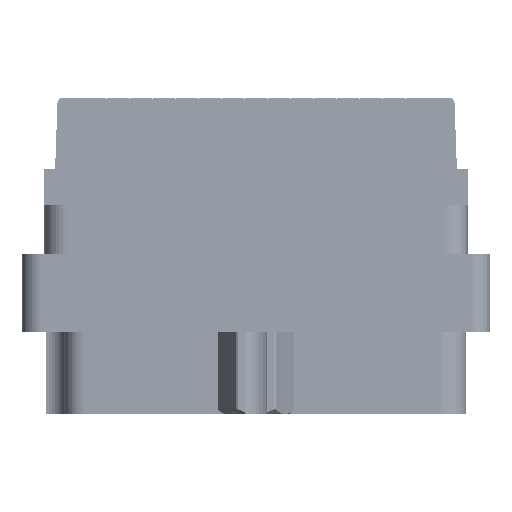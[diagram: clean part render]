
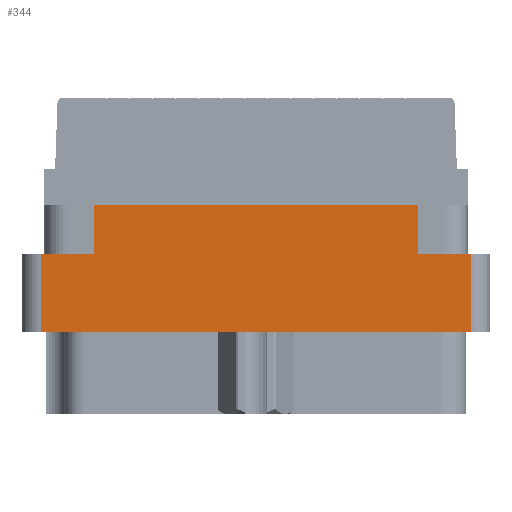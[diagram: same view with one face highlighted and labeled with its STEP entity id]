
A CAD part, left-side view. The second image highlights one B-rep face of the part: STEP entity #344.
In plain terms, the highlighted planar face has unit normal (-1, 0, 0).
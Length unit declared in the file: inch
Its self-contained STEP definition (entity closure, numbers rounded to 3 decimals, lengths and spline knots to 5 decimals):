
#344 = ADVANCED_FACE ( 'NONE', ( #20530 ), #84524, .T. ) ;
#3969 = CARTESIAN_POINT ( 'NONE',  ( -1.375, -0.5285, -0.277 ) ) ;
#5649 = VERTEX_POINT ( 'NONE', #60037 ) ;
#8174 = VECTOR ( 'NONE', #12368, 39.37008 ) ;
#8323 = DIRECTION ( 'NONE',  ( 0., -1., 0. ) ) ;
#12368 = DIRECTION ( 'NONE',  ( 0., 0., 1. ) ) ;
#13965 = VECTOR ( 'NONE', #39157, 39.37008 ) ;
#16378 = ORIENTED_EDGE ( 'NONE', *, *, #23916, .F. ) ;
#17098 = VECTOR ( 'NONE', #32478, 39.37008 ) ;
#17879 = VERTEX_POINT ( 'NONE', #25842 ) ;
#18598 = CARTESIAN_POINT ( 'NONE',  ( -1.375, 0.5285, -0.117 ) ) ;
#18664 = VERTEX_POINT ( 'NONE', #22468 ) ;
#20475 = DIRECTION ( 'NONE',  ( 0., 0., -1. ) ) ;
#20530 = FACE_OUTER_BOUND ( 'NONE', #51721, .T. ) ;
#22468 = CARTESIAN_POINT ( 'NONE',  ( -1.375, 0.7005, -0.277 ) ) ;
#23916 = EDGE_CURVE ( 'NONE', #62617, #17879, #39679, .T. ) ;
#24290 = ORIENTED_EDGE ( 'NONE', *, *, #96346, .F. ) ;
#25127 = LINE ( 'NONE', #63428, #78192 ) ;
#25420 = VECTOR ( 'NONE', #20475, 39.37008 ) ;
#25500 = CARTESIAN_POINT ( 'NONE',  ( -1.375, 0., -0.529 ) ) ;
#25842 = CARTESIAN_POINT ( 'NONE',  ( -1.375, 0.7005, -0.529 ) ) ;
#29017 = ORIENTED_EDGE ( 'NONE', *, *, #82856, .F. ) ;
#30331 = ORIENTED_EDGE ( 'NONE', *, *, #56601, .T. ) ;
#31224 = CARTESIAN_POINT ( 'NONE',  ( -1.375, -0.7005, -0.529 ) ) ;
#32478 = DIRECTION ( 'NONE',  ( 0., 0., 1. ) ) ;
#32791 = LINE ( 'NONE', #49563, #85825 ) ;
#32966 = CARTESIAN_POINT ( 'NONE',  ( -1.375, 0., -0.277 ) ) ;
#34712 = CARTESIAN_POINT ( 'NONE',  ( -1.375, -0.7625, -0.798 ) ) ;
#36149 = ORIENTED_EDGE ( 'NONE', *, *, #62644, .F. ) ;
#38038 = CARTESIAN_POINT ( 'NONE',  ( -1.375, 0., -0.277 ) ) ;
#39157 = DIRECTION ( 'NONE',  ( 0., 1., 0. ) ) ;
#39679 = LINE ( 'NONE', #25500, #13965 ) ;
#42271 = VECTOR ( 'NONE', #93662, 39.37008 ) ;
#42893 = LINE ( 'NONE', #32966, #91348 ) ;
#45050 = VERTEX_POINT ( 'NONE', #92158 ) ;
#46078 = CARTESIAN_POINT ( 'NONE',  ( -1.375, -0.7005, -0.277 ) ) ;
#49563 = CARTESIAN_POINT ( 'NONE',  ( -1.375, -0.7005, -0.798 ) ) ;
#50468 = VERTEX_POINT ( 'NONE', #46078 ) ;
#51478 = DIRECTION ( 'NONE',  ( -1., 0., 0. ) ) ;
#51721 = EDGE_LOOP ( 'NONE', ( #36149, #102020, #16378, #93341, #24290, #30331, #100045, #29017 ) ) ;
#54832 = LINE ( 'NONE', #38038, #42271 ) ;
#56601 = EDGE_CURVE ( 'NONE', #96442, #45050, #83221, .T. ) ;
#59136 = AXIS2_PLACEMENT_3D ( 'NONE', #34712, #51478, #66718 ) ;
#60037 = CARTESIAN_POINT ( 'NONE',  ( -1.375, 0.5285, -0.277 ) ) ;
#62617 = VERTEX_POINT ( 'NONE', #31224 ) ;
#62644 = EDGE_CURVE ( 'NONE', #18664, #5649, #54832, .T. ) ;
#63428 = CARTESIAN_POINT ( 'NONE',  ( -1.375, 0.7625, -0.117 ) ) ;
#66032 = LINE ( 'NONE', #73394, #17098 ) ;
#66718 = DIRECTION ( 'NONE',  ( 0., 0., 1. ) ) ;
#70483 = VERTEX_POINT ( 'NONE', #18598 ) ;
#73366 = DIRECTION ( 'NONE',  ( 0., -1., 0. ) ) ;
#73394 = CARTESIAN_POINT ( 'NONE',  ( -1.375, 0.5285, -0.277 ) ) ;
#75568 = LINE ( 'NONE', #90798, #25420 ) ;
#78192 = VECTOR ( 'NONE', #8323, 39.37008 ) ;
#82529 = EDGE_CURVE ( 'NONE', #18664, #17879, #75568, .T. ) ;
#82856 = EDGE_CURVE ( 'NONE', #5649, #70483, #66032, .T. ) ;
#83221 = LINE ( 'NONE', #3969, #8174 ) ;
#84524 = PLANE ( 'NONE',  #59136 ) ;
#85468 = EDGE_CURVE ( 'NONE', #70483, #45050, #25127, .T. ) ;
#85825 = VECTOR ( 'NONE', #89454, 39.37008 ) ;
#89454 = DIRECTION ( 'NONE',  ( 0., 0., 1. ) ) ;
#90798 = CARTESIAN_POINT ( 'NONE',  ( -1.375, 0.7005, -0.798 ) ) ;
#91348 = VECTOR ( 'NONE', #73366, 39.37008 ) ;
#92158 = CARTESIAN_POINT ( 'NONE',  ( -1.375, -0.5285, -0.117 ) ) ;
#92188 = CARTESIAN_POINT ( 'NONE',  ( -1.375, -0.5285, -0.277 ) ) ;
#93243 = EDGE_CURVE ( 'NONE', #62617, #50468, #32791, .T. ) ;
#93341 = ORIENTED_EDGE ( 'NONE', *, *, #93243, .T. ) ;
#93662 = DIRECTION ( 'NONE',  ( 0., -1., 0. ) ) ;
#96346 = EDGE_CURVE ( 'NONE', #96442, #50468, #42893, .T. ) ;
#96442 = VERTEX_POINT ( 'NONE', #92188 ) ;
#100045 = ORIENTED_EDGE ( 'NONE', *, *, #85468, .F. ) ;
#102020 = ORIENTED_EDGE ( 'NONE', *, *, #82529, .T. ) ;
